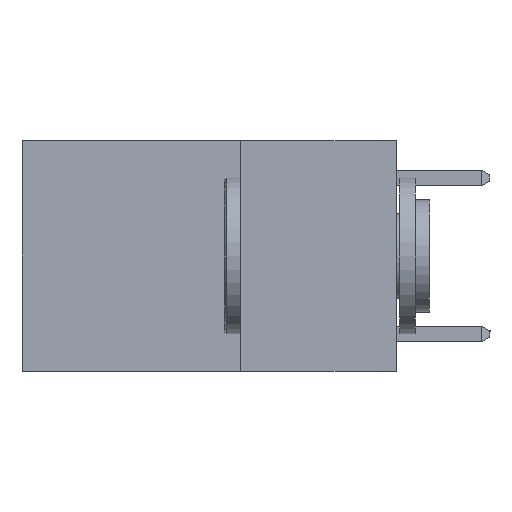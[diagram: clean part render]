
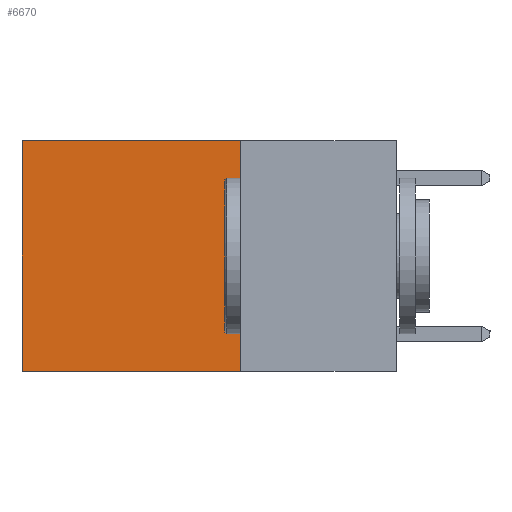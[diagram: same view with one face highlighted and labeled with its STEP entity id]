
A CAD part, left-side view. The second image highlights one B-rep face of the part: STEP entity #6670.
In plain terms, the highlighted planar face has unit normal (-1, 0, 0).
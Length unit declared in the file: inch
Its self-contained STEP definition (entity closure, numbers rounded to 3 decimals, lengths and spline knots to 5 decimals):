
#379 = CARTESIAN_POINT ( 'NONE',  ( 0.2625, 0.25, 0. ) ) ;
#472 = CARTESIAN_POINT ( 'NONE',  ( 0.2625, 0.6, 0. ) ) ;
#1207 = VECTOR ( 'NONE', #1319, 39.37008 ) ;
#1319 = DIRECTION ( 'NONE',  ( 0., 0., -1. ) ) ;
#1493 = LINE ( 'NONE', #379, #1207 ) ;
#1770 = VERTEX_POINT ( 'NONE', #3916 ) ;
#1787 = VECTOR ( 'NONE', #3104, 39.37008 ) ;
#1927 = VECTOR ( 'NONE', #3726, 39.37008 ) ;
#2066 = CARTESIAN_POINT ( 'NONE',  ( 0.2625, 0.25, -0.37 ) ) ;
#2160 = CARTESIAN_POINT ( 'NONE',  ( 0.2625, 0.6, 0. ) ) ;
#2199 = EDGE_LOOP ( 'NONE', ( #10997, #4930, #2269, #6840 ) ) ;
#2269 = ORIENTED_EDGE ( 'NONE', *, *, #7812, .F. ) ;
#2415 = CARTESIAN_POINT ( 'NONE',  ( 0.2625, 0.25, 0. ) ) ;
#2928 = VERTEX_POINT ( 'NONE', #8073 ) ;
#3104 = DIRECTION ( 'NONE',  ( 0., 0., -1. ) ) ;
#3210 = AXIS2_PLACEMENT_3D ( 'NONE', #2415, #4301, #10571 ) ;
#3726 = DIRECTION ( 'NONE',  ( 0., 1., 0. ) ) ;
#3916 = CARTESIAN_POINT ( 'NONE',  ( 0.2625, 0.6, -0.37 ) ) ;
#4213 = VERTEX_POINT ( 'NONE', #472 ) ;
#4301 = DIRECTION ( 'NONE',  ( 1., 0., 0. ) ) ;
#4653 = CARTESIAN_POINT ( 'NONE',  ( 0.2625, 0.25, 0. ) ) ;
#4930 = ORIENTED_EDGE ( 'NONE', *, *, #8509, .F. ) ;
#5687 = LINE ( 'NONE', #2066, #8041 ) ;
#6670 = ADVANCED_FACE ( 'NONE', ( #9268 ), #7006, .F. ) ;
#6712 = DIRECTION ( 'NONE',  ( 0., 1., 0. ) ) ;
#6806 = CARTESIAN_POINT ( 'NONE',  ( 0.2625, 0.25, -0.37 ) ) ;
#6840 = ORIENTED_EDGE ( 'NONE', *, *, #7601, .T. ) ;
#6842 = LINE ( 'NONE', #4653, #1927 ) ;
#6973 = LINE ( 'NONE', #2160, #1787 ) ;
#7006 = PLANE ( 'NONE',  #3210 ) ;
#7601 = EDGE_CURVE ( 'NONE', #2928, #4213, #6842, .T. ) ;
#7789 = EDGE_CURVE ( 'NONE', #4213, #1770, #6973, .T. ) ;
#7802 = VERTEX_POINT ( 'NONE', #6806 ) ;
#7812 = EDGE_CURVE ( 'NONE', #2928, #7802, #1493, .T. ) ;
#8041 = VECTOR ( 'NONE', #6712, 39.37008 ) ;
#8073 = CARTESIAN_POINT ( 'NONE',  ( 0.2625, 0.25, 0. ) ) ;
#8509 = EDGE_CURVE ( 'NONE', #7802, #1770, #5687, .T. ) ;
#9268 = FACE_OUTER_BOUND ( 'NONE', #2199, .T. ) ;
#10571 = DIRECTION ( 'NONE',  ( 0., 0., -1. ) ) ;
#10997 = ORIENTED_EDGE ( 'NONE', *, *, #7789, .T. ) ;
